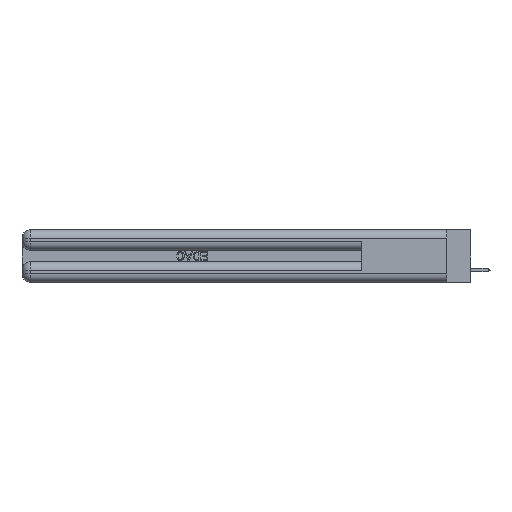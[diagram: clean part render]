
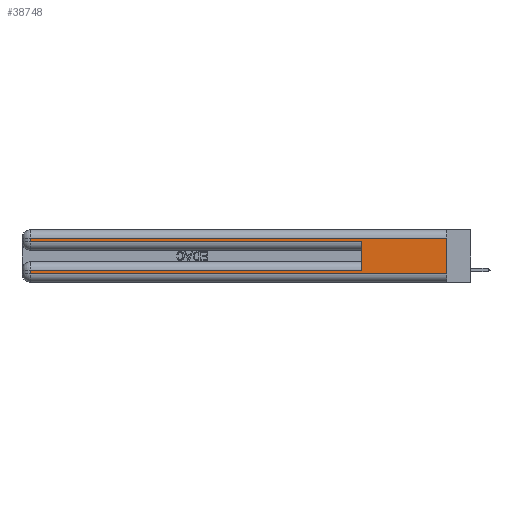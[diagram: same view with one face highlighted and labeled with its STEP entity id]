
A CAD part, left-side view. The second image highlights one B-rep face of the part: STEP entity #38748.
In plain terms, the highlighted planar face has unit normal (-1, 0, 0).
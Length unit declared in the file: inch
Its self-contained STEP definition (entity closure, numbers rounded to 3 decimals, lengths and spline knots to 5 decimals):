
#645 = LINE ( 'NONE', #10526, #8443 ) ;
#1440 = VECTOR ( 'NONE', #4152, 39.37008 ) ;
#2282 = FACE_OUTER_BOUND ( 'NONE', #35408, .T. ) ;
#2985 = VECTOR ( 'NONE', #12807, 39.37008 ) ;
#4152 = DIRECTION ( 'NONE',  ( 0., 0., -1. ) ) ;
#4896 = VERTEX_POINT ( 'NONE', #26307 ) ;
#5875 = CARTESIAN_POINT ( 'NONE',  ( 0., 0., 0.06 ) ) ;
#6350 = CARTESIAN_POINT ( 'NONE',  ( 0., 0., 0.285 ) ) ;
#7024 = CARTESIAN_POINT ( 'NONE',  ( 0., 0., 0.37 ) ) ;
#8443 = VECTOR ( 'NONE', #33127, 39.37008 ) ;
#8528 = EDGE_CURVE ( 'NONE', #43984, #4896, #21747, .T. ) ;
#8953 = VECTOR ( 'NONE', #23202, 39.37008 ) ;
#9684 = DIRECTION ( 'NONE',  ( 0., 0., -1. ) ) ;
#10526 = CARTESIAN_POINT ( 'NONE',  ( 0., 2.94, 0.37 ) ) ;
#12133 = EDGE_CURVE ( 'NONE', #12337, #4896, #20127, .T. ) ;
#12337 = VERTEX_POINT ( 'NONE', #31177 ) ;
#12807 = DIRECTION ( 'NONE',  ( 0., 1., 0. ) ) ;
#13112 = LINE ( 'NONE', #16055, #8953 ) ;
#13617 = ORIENTED_EDGE ( 'NONE', *, *, #39958, .T. ) ;
#14235 = VECTOR ( 'NONE', #40253, 39.37008 ) ;
#16055 = CARTESIAN_POINT ( 'NONE',  ( 0., 0.6, 0.145 ) ) ;
#17124 = VERTEX_POINT ( 'NONE', #40854 ) ;
#17155 = CARTESIAN_POINT ( 'NONE',  ( 0., 0., 0.37 ) ) ;
#17249 = VECTOR ( 'NONE', #26063, 39.37008 ) ;
#19952 = AXIS2_PLACEMENT_3D ( 'NONE', #17155, #32472, #9684 ) ;
#20127 = LINE ( 'NONE', #5875, #14235 ) ;
#21404 = ORIENTED_EDGE ( 'NONE', *, *, #47274, .T. ) ;
#21747 = LINE ( 'NONE', #7024, #1440 ) ;
#22588 = LINE ( 'NONE', #47545, #36312 ) ;
#23202 = DIRECTION ( 'NONE',  ( 0., 0., 1. ) ) ;
#24087 = CARTESIAN_POINT ( 'NONE',  ( 0., 0., 0.31 ) ) ;
#24925 = ORIENTED_EDGE ( 'NONE', *, *, #12133, .T. ) ;
#25364 = ORIENTED_EDGE ( 'NONE', *, *, #41797, .T. ) ;
#26063 = DIRECTION ( 'NONE',  ( 0., 0., -1. ) ) ;
#26242 = CARTESIAN_POINT ( 'NONE',  ( 0., 2.94, 0.37 ) ) ;
#26307 = CARTESIAN_POINT ( 'NONE',  ( 0., 0., 0.06 ) ) ;
#27467 = ORIENTED_EDGE ( 'NONE', *, *, #8528, .F. ) ;
#29348 = ORIENTED_EDGE ( 'NONE', *, *, #37099, .T. ) ;
#30503 = CARTESIAN_POINT ( 'NONE',  ( 0., 2.94, 0.31 ) ) ;
#31177 = CARTESIAN_POINT ( 'NONE',  ( 0., 2.94, 0.06 ) ) ;
#31238 = EDGE_CURVE ( 'NONE', #46428, #17124, #13112, .T. ) ;
#32367 = DIRECTION ( 'NONE',  ( 0., 1., 0. ) ) ;
#32472 = DIRECTION ( 'NONE',  ( 1., 0., 0. ) ) ;
#33127 = DIRECTION ( 'NONE',  ( 0., 0., -1. ) ) ;
#34966 = CARTESIAN_POINT ( 'NONE',  ( 0., 0.6, 0.085 ) ) ;
#35408 = EDGE_LOOP ( 'NONE', ( #27467, #36970, #21404, #13617, #36622, #25364, #29348, #24925 ) ) ;
#36312 = VECTOR ( 'NONE', #32367, 39.37008 ) ;
#36622 = ORIENTED_EDGE ( 'NONE', *, *, #31238, .F. ) ;
#36970 = ORIENTED_EDGE ( 'NONE', *, *, #46925, .T. ) ;
#37099 = EDGE_CURVE ( 'NONE', #40633, #12337, #645, .T. ) ;
#37681 = LINE ( 'NONE', #6350, #46560 ) ;
#37992 = CARTESIAN_POINT ( 'NONE',  ( 0., 0., 0.31 ) ) ;
#38698 = LINE ( 'NONE', #26242, #17249 ) ;
#38748 = ADVANCED_FACE ( 'NONE', ( #2282 ), #40017, .F. ) ;
#39319 = CARTESIAN_POINT ( 'NONE',  ( 0., 2.94, 0.085 ) ) ;
#39933 = VERTEX_POINT ( 'NONE', #30503 ) ;
#39958 = EDGE_CURVE ( 'NONE', #43195, #17124, #37681, .T. ) ;
#40017 = PLANE ( 'NONE',  #19952 ) ;
#40253 = DIRECTION ( 'NONE',  ( 0., -1., 0. ) ) ;
#40633 = VERTEX_POINT ( 'NONE', #39319 ) ;
#40854 = CARTESIAN_POINT ( 'NONE',  ( 0., 0.6, 0.285 ) ) ;
#41797 = EDGE_CURVE ( 'NONE', #46428, #40633, #22588, .T. ) ;
#43195 = VERTEX_POINT ( 'NONE', #48745 ) ;
#43984 = VERTEX_POINT ( 'NONE', #37992 ) ;
#46428 = VERTEX_POINT ( 'NONE', #34966 ) ;
#46560 = VECTOR ( 'NONE', #48511, 39.37008 ) ;
#46925 = EDGE_CURVE ( 'NONE', #43984, #39933, #47699, .T. ) ;
#47274 = EDGE_CURVE ( 'NONE', #39933, #43195, #38698, .T. ) ;
#47545 = CARTESIAN_POINT ( 'NONE',  ( 0., 0., 0.085 ) ) ;
#47699 = LINE ( 'NONE', #24087, #2985 ) ;
#48511 = DIRECTION ( 'NONE',  ( 0., -1., 0. ) ) ;
#48745 = CARTESIAN_POINT ( 'NONE',  ( 0., 2.94, 0.285 ) ) ;
